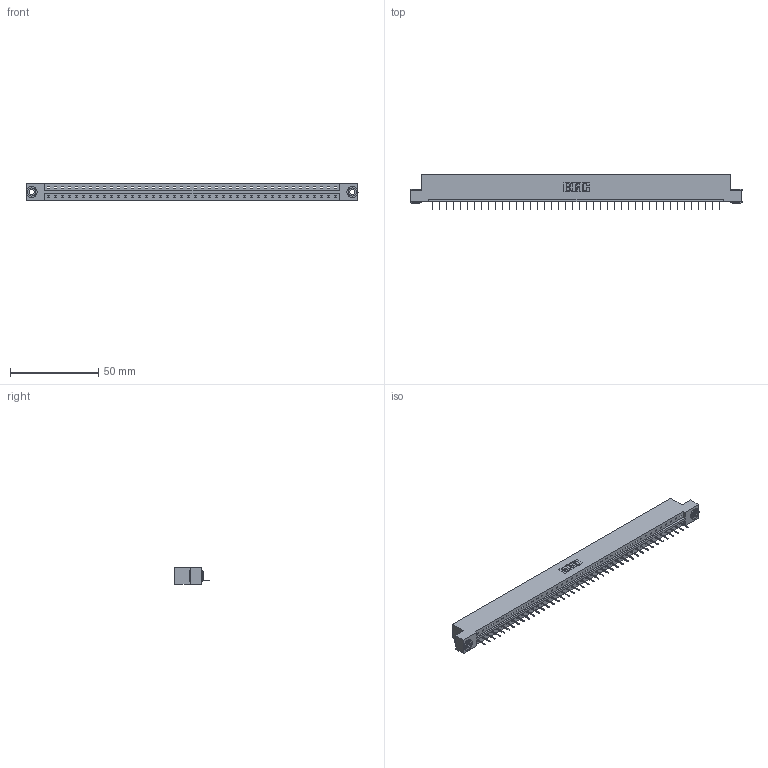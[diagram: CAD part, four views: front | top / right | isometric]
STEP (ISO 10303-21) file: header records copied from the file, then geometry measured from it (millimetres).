
FILE_DESCRIPTION (( 'STEP AP203' ), '1' );
FILE_NAME ('333-042-524-103.STEP', '2018-08-03T18:40:32', ( '' ), ( '' ), 'SwSTEP 2.0', 'SolidWorks 2016', '' );
FILE_SCHEMA (( 'CONFIG_CONTROL_DESIGN' ));
Length unit declared in the file: inch
Products named in the file (4): 333-042-524-103; 333 Part_Flush - .156 Dia - TH; 345-292-001_345-293-124; 345-250-002_345-250-002-102
Assembly tree (45 placements, depth 2):
  333-042-524-103
    333 Part_Flush - .156 Dia - TH
    345-292-001_345-293-124  x42
    345-250-002_345-250-002-102  x2
Bounding box: 187.96 x 19.69 x 9.4 mm (x, y, z)
Volume: 18767.6 mm3; surface area: 19963.6 mm2
Topology: 45 solids, 45 shells, 2756 faces, 7947 edges, 5126 vertices
Faces by surface type: plane 2096, cylinder 652, cone 8
Entity records: 26400 total; most frequent: CARTESIAN_POINT 4531, ORIENTED_EDGE 4502, DIRECTION 3857, EDGE_CURVE 2251, VECTOR 2103, LINE 2103, VERTEX_POINT 1494, AXIS2_PLACEMENT_3D 877
